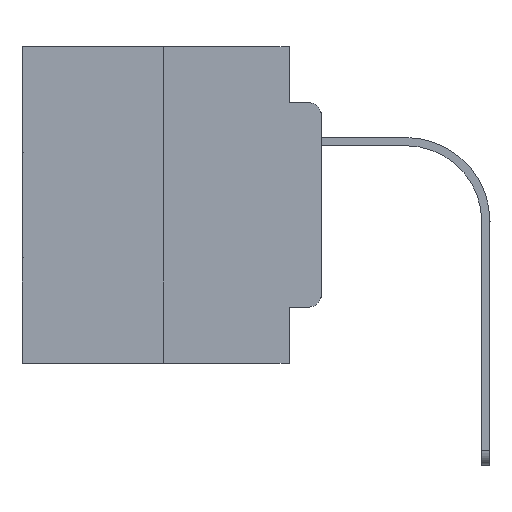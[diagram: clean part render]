
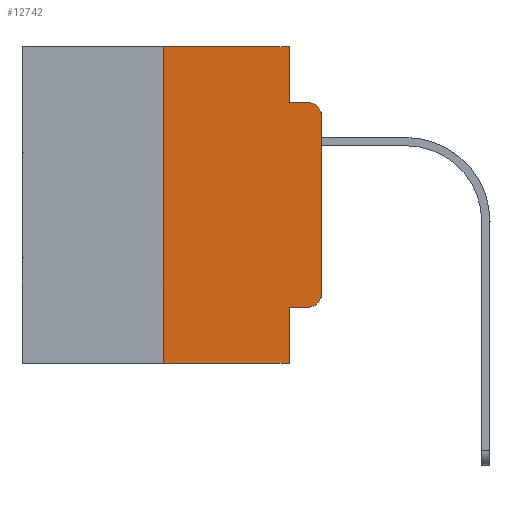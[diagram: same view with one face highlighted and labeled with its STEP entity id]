
A CAD part, left-side view. The second image highlights one B-rep face of the part: STEP entity #12742.
In plain terms, the highlighted planar face has unit normal (-1, 0, 0).
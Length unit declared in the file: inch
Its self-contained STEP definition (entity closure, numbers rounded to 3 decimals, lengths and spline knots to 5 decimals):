
#1287 = DIRECTION ( 'NONE',  ( 0., 0., -1. ) ) ;
#1615 = ORIENTED_EDGE ( 'NONE', *, *, #8253, .F. ) ;
#2125 = LINE ( 'NONE', #8863, #13192 ) ;
#2336 = ORIENTED_EDGE ( 'NONE', *, *, #11819, .T. ) ;
#2878 = ORIENTED_EDGE ( 'NONE', *, *, #20887, .F. ) ;
#3332 = EDGE_CURVE ( 'NONE', #19299, #15210, #21823, .T. ) ;
#3399 = CARTESIAN_POINT ( 'NONE',  ( 0., 0.473, 0. ) ) ;
#3586 = CARTESIAN_POINT ( 'NONE',  ( 0., 0.051, 0. ) ) ;
#3907 = CARTESIAN_POINT ( 'NONE',  ( 0., 0., -0.1085 ) ) ;
#4046 = DIRECTION ( 'NONE',  ( 0., 0., -1. ) ) ;
#4439 = VECTOR ( 'NONE', #8541, 39.37008 ) ;
#4655 = EDGE_CURVE ( 'NONE', #26324, #20040, #21200, .T. ) ;
#4821 = DIRECTION ( 'NONE',  ( 0., 0., 1. ) ) ;
#5219 = VECTOR ( 'NONE', #4821, 39.37008 ) ;
#5511 = CARTESIAN_POINT ( 'NONE',  ( 0., 0.051, -0.5 ) ) ;
#5917 = CARTESIAN_POINT ( 'NONE',  ( 0., 0.02, -0.0885 ) ) ;
#5935 = EDGE_CURVE ( 'NONE', #19299, #15723, #10410, .T. ) ;
#6289 = LINE ( 'NONE', #10775, #4439 ) ;
#6706 = VECTOR ( 'NONE', #20176, 39.37008 ) ;
#6920 = CARTESIAN_POINT ( 'NONE',  ( 0., 0.25, 0. ) ) ;
#7072 = ORIENTED_EDGE ( 'NONE', *, *, #5935, .T. ) ;
#7173 = VECTOR ( 'NONE', #22149, 39.37008 ) ;
#7694 = VERTEX_POINT ( 'NONE', #3586 ) ;
#8130 = VERTEX_POINT ( 'NONE', #5917 ) ;
#8253 = EDGE_CURVE ( 'NONE', #15023, #8130, #2125, .T. ) ;
#8541 = DIRECTION ( 'NONE',  ( 0., 0., 1. ) ) ;
#8592 = DIRECTION ( 'NONE',  ( -1., 0., 0. ) ) ;
#8726 = CARTESIAN_POINT ( 'NONE',  ( 0., 0.473, -0.5 ) ) ;
#8863 = CARTESIAN_POINT ( 'NONE',  ( 0., 0.051, -0.0885 ) ) ;
#9288 = CIRCLE ( 'NONE', #24984, 0.02 ) ;
#9630 = LINE ( 'NONE', #18178, #7173 ) ;
#9763 = ORIENTED_EDGE ( 'NONE', *, *, #25721, .T. ) ;
#9785 = LINE ( 'NONE', #22712, #9868 ) ;
#9817 = DIRECTION ( 'NONE',  ( -1., 0., 0. ) ) ;
#9868 = VECTOR ( 'NONE', #25227, 39.37008 ) ;
#9998 = VECTOR ( 'NONE', #18966, 39.37008 ) ;
#10410 = LINE ( 'NONE', #8726, #9998 ) ;
#10775 = CARTESIAN_POINT ( 'NONE',  ( 0., 0., 0. ) ) ;
#11191 = CARTESIAN_POINT ( 'NONE',  ( 0., 0.473, 0. ) ) ;
#11513 = VERTEX_POINT ( 'NONE', #16384 ) ;
#11819 = EDGE_CURVE ( 'NONE', #21775, #8130, #9288, .T. ) ;
#12014 = EDGE_CURVE ( 'NONE', #7694, #15023, #15119, .T. ) ;
#12202 = CARTESIAN_POINT ( 'NONE',  ( 0., 0.02, -0.1085 ) ) ;
#12742 = ADVANCED_FACE ( 'NONE', ( #14063 ), #22642, .F. ) ;
#12946 = CARTESIAN_POINT ( 'NONE',  ( 0., 0.02, -0.3915 ) ) ;
#13192 = VECTOR ( 'NONE', #21206, 39.37008 ) ;
#13366 = CARTESIAN_POINT ( 'NONE',  ( 0., 0., -0.3915 ) ) ;
#14063 = FACE_OUTER_BOUND ( 'NONE', #14382, .T. ) ;
#14104 = CARTESIAN_POINT ( 'NONE',  ( 0., 0.25, 0. ) ) ;
#14382 = EDGE_LOOP ( 'NONE', ( #26282, #2336, #1615, #18652, #2878, #16143, #7072, #25026, #9763, #18897 ) ) ;
#15023 = VERTEX_POINT ( 'NONE', #18896 ) ;
#15119 = LINE ( 'NONE', #17080, #22702 ) ;
#15210 = VERTEX_POINT ( 'NONE', #14104 ) ;
#15392 = LINE ( 'NONE', #11191, #6706 ) ;
#15723 = VERTEX_POINT ( 'NONE', #5511 ) ;
#16143 = ORIENTED_EDGE ( 'NONE', *, *, #3332, .F. ) ;
#16165 = EDGE_CURVE ( 'NONE', #11513, #15723, #9630, .T. ) ;
#16384 = CARTESIAN_POINT ( 'NONE',  ( 0., 0.051, -0.4115 ) ) ;
#16863 = CARTESIAN_POINT ( 'NONE',  ( 0., 0.25, -0.5 ) ) ;
#17080 = CARTESIAN_POINT ( 'NONE',  ( 0., 0.051, 0. ) ) ;
#17131 = DIRECTION ( 'NONE',  ( 0., 0., -1. ) ) ;
#18178 = CARTESIAN_POINT ( 'NONE',  ( 0., 0.051, 0. ) ) ;
#18652 = ORIENTED_EDGE ( 'NONE', *, *, #12014, .F. ) ;
#18896 = CARTESIAN_POINT ( 'NONE',  ( 0., 0.051, -0.0885 ) ) ;
#18897 = ORIENTED_EDGE ( 'NONE', *, *, #4655, .T. ) ;
#18966 = DIRECTION ( 'NONE',  ( 0., -1., 0. ) ) ;
#19299 = VERTEX_POINT ( 'NONE', #16863 ) ;
#20040 = VERTEX_POINT ( 'NONE', #13366 ) ;
#20176 = DIRECTION ( 'NONE',  ( 0., -1., 0. ) ) ;
#20511 = DIRECTION ( 'NONE',  ( 1., 0., 0. ) ) ;
#20887 = EDGE_CURVE ( 'NONE', #15210, #7694, #15392, .T. ) ;
#21200 = CIRCLE ( 'NONE', #23469, 0.02 ) ;
#21206 = DIRECTION ( 'NONE',  ( 0., -1., 0. ) ) ;
#21352 = AXIS2_PLACEMENT_3D ( 'NONE', #3399, #20511, #1287 ) ;
#21775 = VERTEX_POINT ( 'NONE', #3907 ) ;
#21823 = LINE ( 'NONE', #6920, #5219 ) ;
#22052 = EDGE_CURVE ( 'NONE', #20040, #21775, #6289, .T. ) ;
#22149 = DIRECTION ( 'NONE',  ( 0., 0., -1. ) ) ;
#22642 = PLANE ( 'NONE',  #21352 ) ;
#22702 = VECTOR ( 'NONE', #4046, 39.37008 ) ;
#22712 = CARTESIAN_POINT ( 'NONE',  ( 0., 0.051, -0.4115 ) ) ;
#22747 = DIRECTION ( 'NONE',  ( 0., 0., -1. ) ) ;
#23469 = AXIS2_PLACEMENT_3D ( 'NONE', #12946, #8592, #17131 ) ;
#23492 = CARTESIAN_POINT ( 'NONE',  ( 0., 0.02, -0.4115 ) ) ;
#24984 = AXIS2_PLACEMENT_3D ( 'NONE', #12202, #9817, #22747 ) ;
#25026 = ORIENTED_EDGE ( 'NONE', *, *, #16165, .F. ) ;
#25227 = DIRECTION ( 'NONE',  ( 0., -1., 0. ) ) ;
#25721 = EDGE_CURVE ( 'NONE', #11513, #26324, #9785, .T. ) ;
#26282 = ORIENTED_EDGE ( 'NONE', *, *, #22052, .T. ) ;
#26324 = VERTEX_POINT ( 'NONE', #23492 ) ;
